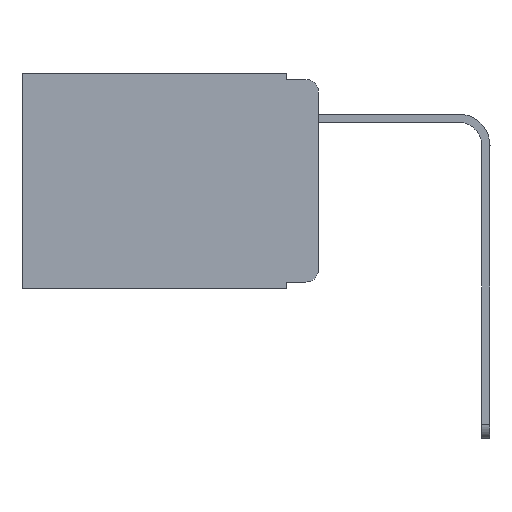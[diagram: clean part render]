
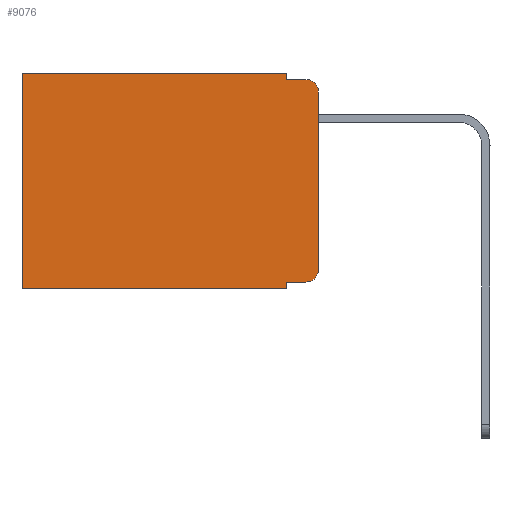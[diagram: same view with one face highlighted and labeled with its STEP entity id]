
A CAD part, left-side view. The second image highlights one B-rep face of the part: STEP entity #9076.
In plain terms, the highlighted planar face has unit normal (-1, 0, 0).
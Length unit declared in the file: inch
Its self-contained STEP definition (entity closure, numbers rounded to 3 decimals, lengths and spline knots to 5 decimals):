
#210 = DIRECTION ( 'NONE',  ( 0., 0., -1. ) ) ;
#257 = DIRECTION ( 'NONE',  ( 0., -1., 0. ) ) ;
#328 = EDGE_CURVE ( 'NONE', #1471, #4284, #9192, .T. ) ;
#852 = VECTOR ( 'NONE', #11212, 39.37008 ) ;
#1065 = CARTESIAN_POINT ( 'NONE',  ( 0.298, 0., -0.03 ) ) ;
#1096 = CARTESIAN_POINT ( 'NONE',  ( 0.298, 0.051, -0.343 ) ) ;
#1382 = VECTOR ( 'NONE', #8790, 39.37008 ) ;
#1414 = CARTESIAN_POINT ( 'NONE',  ( 0.298, 0., -0.313 ) ) ;
#1471 = VERTEX_POINT ( 'NONE', #2850 ) ;
#1485 = AXIS2_PLACEMENT_3D ( 'NONE', #8192, #3219, #12491 ) ;
#1714 = FACE_OUTER_BOUND ( 'NONE', #9159, .T. ) ;
#1758 = CARTESIAN_POINT ( 'NONE',  ( 0.298, 0., 0. ) ) ;
#1872 = VECTOR ( 'NONE', #210, 39.37008 ) ;
#2003 = CIRCLE ( 'NONE', #2095, 0.02 ) ;
#2034 = CARTESIAN_POINT ( 'NONE',  ( 0.298, 0.051, 0. ) ) ;
#2095 = AXIS2_PLACEMENT_3D ( 'NONE', #5411, #8330, #8417 ) ;
#2601 = DIRECTION ( 'NONE',  ( 0., 0., -1. ) ) ;
#2682 = CARTESIAN_POINT ( 'NONE',  ( 0.298, 0.473, 0. ) ) ;
#2850 = CARTESIAN_POINT ( 'NONE',  ( 0.298, 0.051, 0. ) ) ;
#3035 = ORIENTED_EDGE ( 'NONE', *, *, #12262, .T. ) ;
#3162 = CARTESIAN_POINT ( 'NONE',  ( 0.298, 0.473, 0. ) ) ;
#3219 = DIRECTION ( 'NONE',  ( 1., 0., 0. ) ) ;
#3533 = LINE ( 'NONE', #1758, #11294 ) ;
#3596 = VERTEX_POINT ( 'NONE', #4895 ) ;
#3686 = LINE ( 'NONE', #2034, #5753 ) ;
#3760 = ORIENTED_EDGE ( 'NONE', *, *, #4837, .T. ) ;
#3834 = CARTESIAN_POINT ( 'NONE',  ( 0.298, 0., 0. ) ) ;
#4149 = VERTEX_POINT ( 'NONE', #4282 ) ;
#4282 = CARTESIAN_POINT ( 'NONE',  ( 0.298, 0.473, -0.343 ) ) ;
#4284 = VERTEX_POINT ( 'NONE', #7717 ) ;
#4731 = CARTESIAN_POINT ( 'NONE',  ( 0.298, 0.051, -0.01 ) ) ;
#4837 = EDGE_CURVE ( 'NONE', #3596, #11090, #13019, .T. ) ;
#4895 = CARTESIAN_POINT ( 'NONE',  ( 0.298, 0.051, -0.333 ) ) ;
#5411 = CARTESIAN_POINT ( 'NONE',  ( 0.298, 0.02, -0.313 ) ) ;
#5753 = VECTOR ( 'NONE', #7124, 39.37008 ) ;
#5876 = VERTEX_POINT ( 'NONE', #1065 ) ;
#6158 = EDGE_CURVE ( 'NONE', #1471, #6974, #6567, .T. ) ;
#6179 = PLANE ( 'NONE',  #1485 ) ;
#6251 = CARTESIAN_POINT ( 'NONE',  ( 0.298, 0.051, 0. ) ) ;
#6461 = CARTESIAN_POINT ( 'NONE',  ( 0.298, 0.051, -0.333 ) ) ;
#6567 = LINE ( 'NONE', #3834, #7682 ) ;
#6656 = DIRECTION ( 'NONE',  ( -1., 0., 0. ) ) ;
#6706 = ORIENTED_EDGE ( 'NONE', *, *, #11041, .T. ) ;
#6745 = LINE ( 'NONE', #10080, #9412 ) ;
#6974 = VERTEX_POINT ( 'NONE', #2682 ) ;
#7002 = ORIENTED_EDGE ( 'NONE', *, *, #328, .F. ) ;
#7120 = DIRECTION ( 'NONE',  ( 0., 1., 0. ) ) ;
#7124 = DIRECTION ( 'NONE',  ( 0., 0., -1. ) ) ;
#7191 = CARTESIAN_POINT ( 'NONE',  ( 0.298, 0.02, -0.03 ) ) ;
#7396 = ORIENTED_EDGE ( 'NONE', *, *, #8527, .F. ) ;
#7503 = EDGE_CURVE ( 'NONE', #5876, #11883, #3533, .T. ) ;
#7682 = VECTOR ( 'NONE', #11892, 39.37008 ) ;
#7717 = CARTESIAN_POINT ( 'NONE',  ( 0.298, 0.051, -0.01 ) ) ;
#7812 = LINE ( 'NONE', #4731, #1382 ) ;
#7840 = EDGE_CURVE ( 'NONE', #3596, #11807, #3686, .T. ) ;
#7980 = ORIENTED_EDGE ( 'NONE', *, *, #10311, .T. ) ;
#8192 = CARTESIAN_POINT ( 'NONE',  ( 0.298, 0., 0. ) ) ;
#8330 = DIRECTION ( 'NONE',  ( -1., 0., 0. ) ) ;
#8417 = DIRECTION ( 'NONE',  ( 0., 0., -1. ) ) ;
#8527 = EDGE_CURVE ( 'NONE', #11807, #4149, #6745, .T. ) ;
#8790 = DIRECTION ( 'NONE',  ( 0., -1., 0. ) ) ;
#8899 = ORIENTED_EDGE ( 'NONE', *, *, #10619, .F. ) ;
#9076 = ADVANCED_FACE ( 'NONE', ( #1714 ), #6179, .F. ) ;
#9159 = EDGE_LOOP ( 'NONE', ( #10421, #7980, #8899, #7002, #10480, #3035, #7396, #11014, #3760, #6706 ) ) ;
#9192 = LINE ( 'NONE', #6251, #852 ) ;
#9412 = VECTOR ( 'NONE', #7120, 39.37008 ) ;
#9732 = CARTESIAN_POINT ( 'NONE',  ( 0.298, 0.02, -0.01 ) ) ;
#10080 = CARTESIAN_POINT ( 'NONE',  ( 0.298, 0., -0.343 ) ) ;
#10311 = EDGE_CURVE ( 'NONE', #5876, #12046, #12419, .T. ) ;
#10421 = ORIENTED_EDGE ( 'NONE', *, *, #7503, .F. ) ;
#10480 = ORIENTED_EDGE ( 'NONE', *, *, #6158, .T. ) ;
#10619 = EDGE_CURVE ( 'NONE', #4284, #12046, #7812, .T. ) ;
#10732 = LINE ( 'NONE', #3162, #1872 ) ;
#11009 = DIRECTION ( 'NONE',  ( 0., 0., -1. ) ) ;
#11014 = ORIENTED_EDGE ( 'NONE', *, *, #7840, .F. ) ;
#11041 = EDGE_CURVE ( 'NONE', #11090, #11883, #2003, .T. ) ;
#11090 = VERTEX_POINT ( 'NONE', #12359 ) ;
#11212 = DIRECTION ( 'NONE',  ( 0., 0., -1. ) ) ;
#11294 = VECTOR ( 'NONE', #2601, 39.37008 ) ;
#11444 = VECTOR ( 'NONE', #257, 39.37008 ) ;
#11807 = VERTEX_POINT ( 'NONE', #1096 ) ;
#11883 = VERTEX_POINT ( 'NONE', #1414 ) ;
#11892 = DIRECTION ( 'NONE',  ( 0., 1., 0. ) ) ;
#12046 = VERTEX_POINT ( 'NONE', #9732 ) ;
#12262 = EDGE_CURVE ( 'NONE', #6974, #4149, #10732, .T. ) ;
#12359 = CARTESIAN_POINT ( 'NONE',  ( 0.298, 0.02, -0.333 ) ) ;
#12419 = CIRCLE ( 'NONE', #13009, 0.02 ) ;
#12491 = DIRECTION ( 'NONE',  ( 0., 0., -1. ) ) ;
#13009 = AXIS2_PLACEMENT_3D ( 'NONE', #7191, #6656, #11009 ) ;
#13019 = LINE ( 'NONE', #6461, #11444 ) ;
